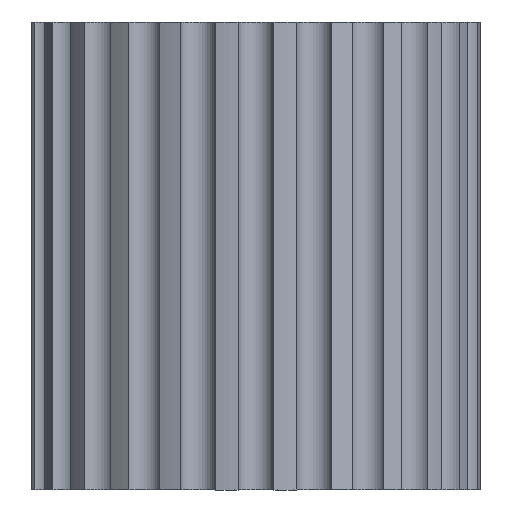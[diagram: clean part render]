
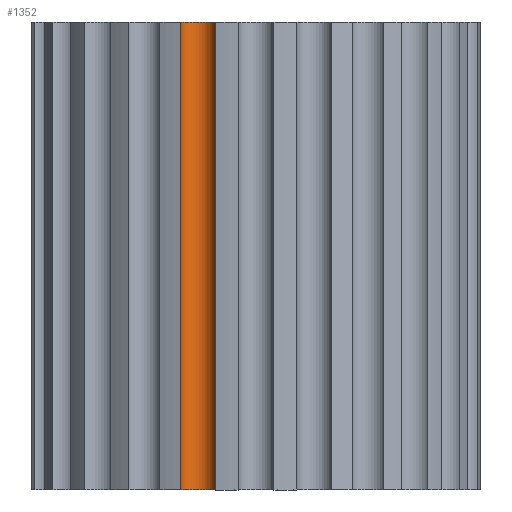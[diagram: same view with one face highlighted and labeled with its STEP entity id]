
A CAD part, front view. The second image highlights one B-rep face of the part: STEP entity #1352.
In plain terms, the highlighted cylindrical face has radius 0.635 mm (diameter 1.27 mm), a partial arc.
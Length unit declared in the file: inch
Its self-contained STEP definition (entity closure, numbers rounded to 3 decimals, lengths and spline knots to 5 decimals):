
#40 = VERTEX_POINT ( 'NONE', #3256 ) ;
#428 = EDGE_LOOP ( 'NONE', ( #469, #6726, #602, #1274 ) ) ;
#469 = ORIENTED_EDGE ( 'NONE', *, *, #6253, .F. ) ;
#602 = ORIENTED_EDGE ( 'NONE', *, *, #6071, .T. ) ;
#885 = DIRECTION ( 'NONE',  ( 0., 0., -1. ) ) ;
#1274 = ORIENTED_EDGE ( 'NONE', *, *, #1805, .T. ) ;
#1314 = LINE ( 'NONE', #1344, #1392 ) ;
#1344 = CARTESIAN_POINT ( 'NONE',  ( -0.10475, -0.29442, -0.01738 ) ) ;
#1352 = ADVANCED_FACE ( 'NONE', ( #5368 ), #1815, .F. ) ;
#1392 = VECTOR ( 'NONE', #885, 39.37008 ) ;
#1564 = VECTOR ( 'NONE', #3779, 39.37008 ) ;
#1694 = AXIS2_PLACEMENT_3D ( 'NONE', #4433, #3369, #3346 ) ;
#1805 = EDGE_CURVE ( 'NONE', #5881, #2307, #1314, .T. ) ;
#1815 = CYLINDRICAL_SURFACE ( 'NONE', #5033, 0.025 ) ;
#2307 = VERTEX_POINT ( 'NONE', #4415 ) ;
#2780 = CARTESIAN_POINT ( 'NONE',  ( -0.05588, -0.30185, -0.23722 ) ) ;
#2875 = LINE ( 'NONE', #2780, #1564 ) ;
#3097 = DIRECTION ( 'NONE',  ( 0., 0., 1. ) ) ;
#3125 = CARTESIAN_POINT ( 'NONE',  ( -0.08088, -0.30185, 0.18259 ) ) ;
#3256 = CARTESIAN_POINT ( 'NONE',  ( -0.05588, -0.30185, 0.18259 ) ) ;
#3344 = DIRECTION ( 'NONE',  ( 1., 0., 0. ) ) ;
#3346 = DIRECTION ( 'NONE',  ( 0., 1., 0. ) ) ;
#3369 = DIRECTION ( 'NONE',  ( 0., 0., 1. ) ) ;
#3692 = EDGE_CURVE ( 'NONE', #4837, #40, #2875, .T. ) ;
#3779 = DIRECTION ( 'NONE',  ( 0., 0., 1. ) ) ;
#3998 = CARTESIAN_POINT ( 'NONE',  ( -0.05588, -0.30185, -0.46741 ) ) ;
#4039 = AXIS2_PLACEMENT_3D ( 'NONE', #3125, #3097, #4162 ) ;
#4162 = DIRECTION ( 'NONE',  ( 1., 0., 0. ) ) ;
#4415 = CARTESIAN_POINT ( 'NONE',  ( -0.10475, -0.29442, -0.46741 ) ) ;
#4433 = CARTESIAN_POINT ( 'NONE',  ( -0.08088, -0.30185, -0.46741 ) ) ;
#4837 = VERTEX_POINT ( 'NONE', #3998 ) ;
#5033 = AXIS2_PLACEMENT_3D ( 'NONE', #5405, #6540, #3344 ) ;
#5109 = CARTESIAN_POINT ( 'NONE',  ( -0.10475, -0.29442, 0.18259 ) ) ;
#5368 = FACE_OUTER_BOUND ( 'NONE', #428, .T. ) ;
#5405 = CARTESIAN_POINT ( 'NONE',  ( -0.08088, -0.30185, -0.23722 ) ) ;
#5856 = CIRCLE ( 'NONE', #4039, 0.025 ) ;
#5881 = VERTEX_POINT ( 'NONE', #5109 ) ;
#6071 = EDGE_CURVE ( 'NONE', #40, #5881, #5856, .T. ) ;
#6196 = CIRCLE ( 'NONE', #1694, 0.025 ) ;
#6253 = EDGE_CURVE ( 'NONE', #4837, #2307, #6196, .T. ) ;
#6540 = DIRECTION ( 'NONE',  ( 0., 0., 1. ) ) ;
#6726 = ORIENTED_EDGE ( 'NONE', *, *, #3692, .T. ) ;
